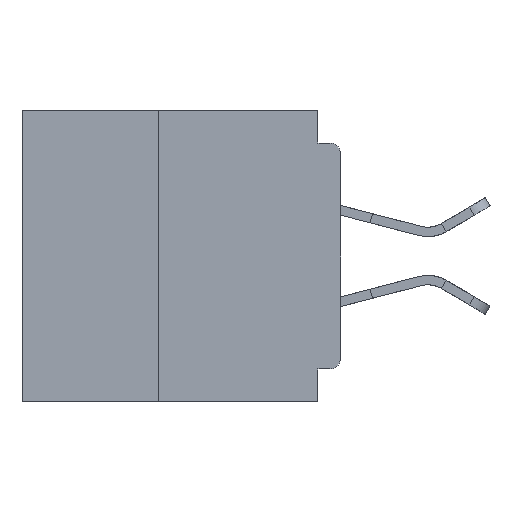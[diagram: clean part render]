
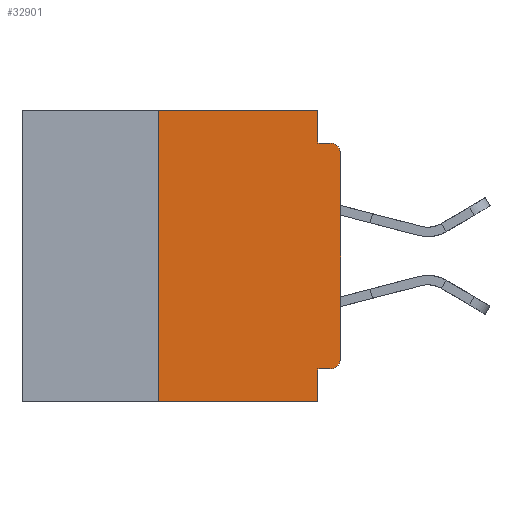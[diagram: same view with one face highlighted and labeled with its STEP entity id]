
A CAD part, left-side view. The second image highlights one B-rep face of the part: STEP entity #32901.
In plain terms, the highlighted planar face has unit normal (-1, 0, 0).
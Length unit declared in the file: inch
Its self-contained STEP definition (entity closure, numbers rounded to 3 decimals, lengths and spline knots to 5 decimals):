
#227 = EDGE_CURVE ( 'NONE', #36416, #2056, #32766, .T. ) ;
#636 = CIRCLE ( 'NONE', #2554, 0.015 ) ;
#915 = EDGE_CURVE ( 'NONE', #36416, #24641, #3768, .T. ) ;
#1216 = CARTESIAN_POINT ( 'NONE',  ( 0., 0.031, 0. ) ) ;
#1992 = EDGE_CURVE ( 'NONE', #30525, #35238, #18920, .T. ) ;
#2056 = VERTEX_POINT ( 'NONE', #21772 ) ;
#2169 = DIRECTION ( 'NONE',  ( 0., 1., 0. ) ) ;
#2554 = AXIS2_PLACEMENT_3D ( 'NONE', #7200, #32014, #10761 ) ;
#2853 = CARTESIAN_POINT ( 'NONE',  ( 0., 0.437, -0.4 ) ) ;
#3031 = EDGE_CURVE ( 'NONE', #2056, #33268, #20459, .T. ) ;
#3692 = CARTESIAN_POINT ( 'NONE',  ( 0., 0., -0.34 ) ) ;
#3768 = LINE ( 'NONE', #2853, #23864 ) ;
#4408 = VECTOR ( 'NONE', #6118, 39.37008 ) ;
#4443 = CARTESIAN_POINT ( 'NONE',  ( 0., 0.031, -0.355 ) ) ;
#5733 = ORIENTED_EDGE ( 'NONE', *, *, #24399, .T. ) ;
#6118 = DIRECTION ( 'NONE',  ( 0., 0., 1. ) ) ;
#6295 = CARTESIAN_POINT ( 'NONE',  ( 0., 0.437, 0. ) ) ;
#6420 = EDGE_CURVE ( 'NONE', #36723, #24641, #7394, .T. ) ;
#7200 = CARTESIAN_POINT ( 'NONE',  ( 0., 0.015, -0.34 ) ) ;
#7394 = LINE ( 'NONE', #30352, #26284 ) ;
#9076 = DIRECTION ( 'NONE',  ( 0., 0., -1. ) ) ;
#9216 = CARTESIAN_POINT ( 'NONE',  ( 0., 0., -0.355 ) ) ;
#9318 = ORIENTED_EDGE ( 'NONE', *, *, #43836, .F. ) ;
#9910 = CARTESIAN_POINT ( 'NONE',  ( 0., 0.015, -0.045 ) ) ;
#9966 = CARTESIAN_POINT ( 'NONE',  ( 0., 0., -0.045 ) ) ;
#10040 = ORIENTED_EDGE ( 'NONE', *, *, #27920, .T. ) ;
#10761 = DIRECTION ( 'NONE',  ( 0., 0., -1. ) ) ;
#11004 = VERTEX_POINT ( 'NONE', #3692 ) ;
#12061 = CARTESIAN_POINT ( 'NONE',  ( 0., 0., 0. ) ) ;
#12211 = DIRECTION ( 'NONE',  ( -1., 0., 0. ) ) ;
#12575 = CARTESIAN_POINT ( 'NONE',  ( 0., 0.015, -0.355 ) ) ;
#13767 = VERTEX_POINT ( 'NONE', #12575 ) ;
#14098 = DIRECTION ( 'NONE',  ( 0., -1., 0. ) ) ;
#14248 = LINE ( 'NONE', #12061, #31970 ) ;
#16513 = CARTESIAN_POINT ( 'NONE',  ( 0., 0.25, -0.4 ) ) ;
#17242 = DIRECTION ( 'NONE',  ( 0., -1., 0. ) ) ;
#18217 = VECTOR ( 'NONE', #22276, 39.37008 ) ;
#18920 = LINE ( 'NONE', #9966, #36612 ) ;
#19160 = CARTESIAN_POINT ( 'NONE',  ( 0., 0.031, -0.4 ) ) ;
#19199 = DIRECTION ( 'NONE',  ( 0., 0., 1. ) ) ;
#20459 = LINE ( 'NONE', #35296, #29891 ) ;
#20613 = DIRECTION ( 'NONE',  ( 1., 0., 0. ) ) ;
#21530 = ORIENTED_EDGE ( 'NONE', *, *, #227, .F. ) ;
#21772 = CARTESIAN_POINT ( 'NONE',  ( 0., 0.25, 0. ) ) ;
#22017 = CARTESIAN_POINT ( 'NONE',  ( 0., 0.031, -0.045 ) ) ;
#22276 = DIRECTION ( 'NONE',  ( 0., 0., -1. ) ) ;
#22502 = CIRCLE ( 'NONE', #27471, 0.015 ) ;
#23390 = ORIENTED_EDGE ( 'NONE', *, *, #3031, .F. ) ;
#23864 = VECTOR ( 'NONE', #17242, 39.37008 ) ;
#24399 = EDGE_CURVE ( 'NONE', #13767, #11004, #636, .T. ) ;
#24641 = VERTEX_POINT ( 'NONE', #19160 ) ;
#26284 = VECTOR ( 'NONE', #9076, 39.37008 ) ;
#27471 = AXIS2_PLACEMENT_3D ( 'NONE', #33417, #12211, #36986 ) ;
#27920 = EDGE_CURVE ( 'NONE', #11004, #43263, #14248, .T. ) ;
#28616 = ORIENTED_EDGE ( 'NONE', *, *, #915, .T. ) ;
#28782 = EDGE_LOOP ( 'NONE', ( #10040, #41204, #37373, #40404, #23390, #21530, #28616, #40998, #9318, #5733 ) ) ;
#28874 = VECTOR ( 'NONE', #2169, 39.37008 ) ;
#29872 = LINE ( 'NONE', #1216, #18217 ) ;
#29891 = VECTOR ( 'NONE', #36020, 39.37008 ) ;
#30352 = CARTESIAN_POINT ( 'NONE',  ( 0., 0.031, -0.4 ) ) ;
#30525 = VERTEX_POINT ( 'NONE', #22017 ) ;
#30533 = CARTESIAN_POINT ( 'NONE',  ( 0., 0., -0.06 ) ) ;
#31127 = PLANE ( 'NONE',  #35575 ) ;
#31970 = VECTOR ( 'NONE', #19199, 39.37008 ) ;
#32014 = DIRECTION ( 'NONE',  ( -1., 0., 0. ) ) ;
#32766 = LINE ( 'NONE', #36260, #4408 ) ;
#32901 = ADVANCED_FACE ( 'NONE', ( #35345 ), #31127, .F. ) ;
#33268 = VERTEX_POINT ( 'NONE', #36662 ) ;
#33417 = CARTESIAN_POINT ( 'NONE',  ( 0., 0.015, -0.06 ) ) ;
#35238 = VERTEX_POINT ( 'NONE', #9910 ) ;
#35296 = CARTESIAN_POINT ( 'NONE',  ( 0., 0.437, 0. ) ) ;
#35345 = FACE_OUTER_BOUND ( 'NONE', #28782, .T. ) ;
#35575 = AXIS2_PLACEMENT_3D ( 'NONE', #6295, #20613, #45277 ) ;
#36020 = DIRECTION ( 'NONE',  ( 0., -1., 0. ) ) ;
#36260 = CARTESIAN_POINT ( 'NONE',  ( 0., 0.25, -0.4 ) ) ;
#36416 = VERTEX_POINT ( 'NONE', #16513 ) ;
#36612 = VECTOR ( 'NONE', #14098, 39.37008 ) ;
#36662 = CARTESIAN_POINT ( 'NONE',  ( 0., 0.031, 0. ) ) ;
#36723 = VERTEX_POINT ( 'NONE', #4443 ) ;
#36986 = DIRECTION ( 'NONE',  ( 0., 0., -1. ) ) ;
#37373 = ORIENTED_EDGE ( 'NONE', *, *, #1992, .F. ) ;
#38265 = LINE ( 'NONE', #9216, #28874 ) ;
#40220 = EDGE_CURVE ( 'NONE', #43263, #35238, #22502, .T. ) ;
#40404 = ORIENTED_EDGE ( 'NONE', *, *, #45570, .F. ) ;
#40998 = ORIENTED_EDGE ( 'NONE', *, *, #6420, .F. ) ;
#41204 = ORIENTED_EDGE ( 'NONE', *, *, #40220, .T. ) ;
#43263 = VERTEX_POINT ( 'NONE', #30533 ) ;
#43836 = EDGE_CURVE ( 'NONE', #13767, #36723, #38265, .T. ) ;
#45277 = DIRECTION ( 'NONE',  ( 0., 0., -1. ) ) ;
#45570 = EDGE_CURVE ( 'NONE', #33268, #30525, #29872, .T. ) ;
